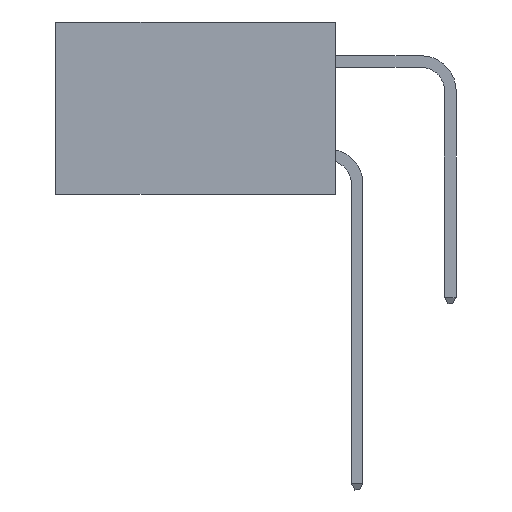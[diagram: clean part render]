
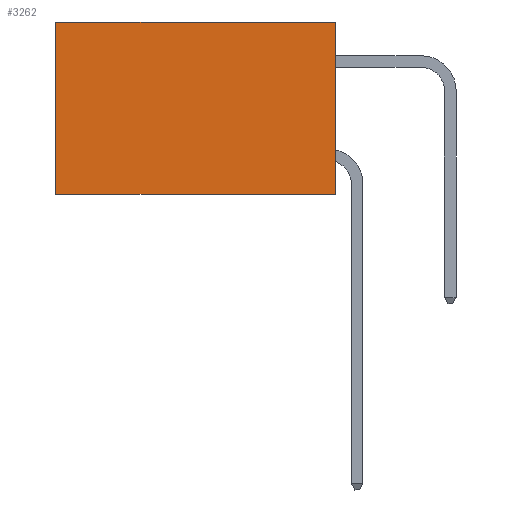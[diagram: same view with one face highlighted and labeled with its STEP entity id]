
A CAD part, left-side view. The second image highlights one B-rep face of the part: STEP entity #3262.
In plain terms, the highlighted planar face has unit normal (-1, 0, 0).
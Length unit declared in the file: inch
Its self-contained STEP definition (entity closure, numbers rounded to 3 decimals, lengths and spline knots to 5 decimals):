
#1379 = ORIENTED_EDGE ( 'NONE', *, *, #17834, .T. ) ;
#2217 = CARTESIAN_POINT ( 'NONE',  ( 0.2875, 0., -0.37 ) ) ;
#2235 = DIRECTION ( 'NONE',  ( 0., 0., -1. ) ) ;
#2488 = VECTOR ( 'NONE', #16003, 39.37008 ) ;
#3133 = CARTESIAN_POINT ( 'NONE',  ( 0.2875, 0.6, 0. ) ) ;
#3213 = CARTESIAN_POINT ( 'NONE',  ( 0.2875, 0., -0.37 ) ) ;
#3262 = ADVANCED_FACE ( 'NONE', ( #22347 ), #18897, .F. ) ;
#3279 = CARTESIAN_POINT ( 'NONE',  ( 0.2875, 0., 0. ) ) ;
#3345 = CARTESIAN_POINT ( 'NONE',  ( 0.2875, 0.6, 0. ) ) ;
#3577 = VERTEX_POINT ( 'NONE', #15020 ) ;
#4210 = CARTESIAN_POINT ( 'NONE',  ( 0.2875, 0., 0. ) ) ;
#7559 = VERTEX_POINT ( 'NONE', #3345 ) ;
#8209 = VERTEX_POINT ( 'NONE', #19637 ) ;
#9403 = DIRECTION ( 'NONE',  ( 0., 0., -1. ) ) ;
#9963 = LINE ( 'NONE', #3213, #13197 ) ;
#10291 = VECTOR ( 'NONE', #9403, 39.37008 ) ;
#11289 = EDGE_LOOP ( 'NONE', ( #13095, #13060, #16252, #1379 ) ) ;
#12955 = VECTOR ( 'NONE', #18595, 39.37008 ) ;
#13060 = ORIENTED_EDGE ( 'NONE', *, *, #25757, .F. ) ;
#13095 = ORIENTED_EDGE ( 'NONE', *, *, #15708, .T. ) ;
#13197 = VECTOR ( 'NONE', #21789, 39.37008 ) ;
#14155 = LINE ( 'NONE', #3133, #10291 ) ;
#15020 = CARTESIAN_POINT ( 'NONE',  ( 0.2875, 0.6, -0.37 ) ) ;
#15708 = EDGE_CURVE ( 'NONE', #7559, #3577, #14155, .T. ) ;
#16003 = DIRECTION ( 'NONE',  ( 0., 1., 0. ) ) ;
#16080 = CARTESIAN_POINT ( 'NONE',  ( 0.2875, 0., 0. ) ) ;
#16252 = ORIENTED_EDGE ( 'NONE', *, *, #21109, .F. ) ;
#17834 = EDGE_CURVE ( 'NONE', #8209, #7559, #22984, .T. ) ;
#18595 = DIRECTION ( 'NONE',  ( 0., 0., -1. ) ) ;
#18897 = PLANE ( 'NONE',  #21646 ) ;
#18925 = DIRECTION ( 'NONE',  ( 1., 0., 0. ) ) ;
#19637 = CARTESIAN_POINT ( 'NONE',  ( 0.2875, 0., 0. ) ) ;
#20577 = VERTEX_POINT ( 'NONE', #2217 ) ;
#21109 = EDGE_CURVE ( 'NONE', #8209, #20577, #26431, .T. ) ;
#21646 = AXIS2_PLACEMENT_3D ( 'NONE', #3279, #18925, #2235 ) ;
#21789 = DIRECTION ( 'NONE',  ( 0., 1., 0. ) ) ;
#22347 = FACE_OUTER_BOUND ( 'NONE', #11289, .T. ) ;
#22984 = LINE ( 'NONE', #16080, #2488 ) ;
#25757 = EDGE_CURVE ( 'NONE', #20577, #3577, #9963, .T. ) ;
#26431 = LINE ( 'NONE', #4210, #12955 ) ;
